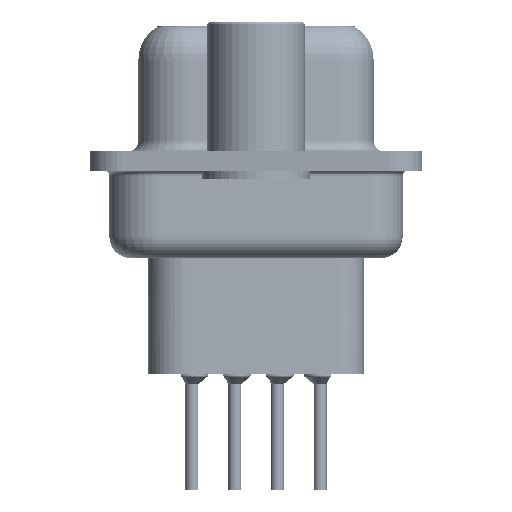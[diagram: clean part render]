
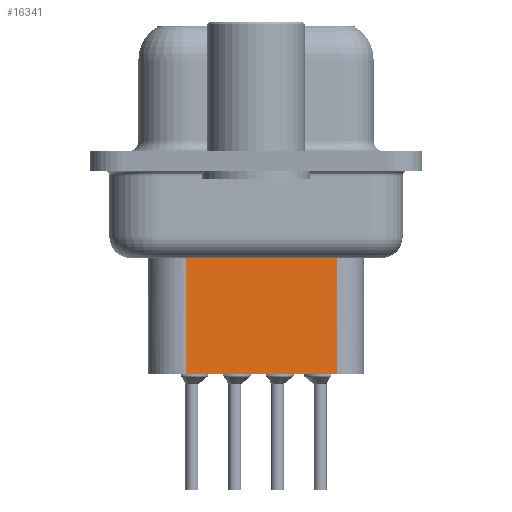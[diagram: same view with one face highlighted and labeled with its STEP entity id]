
A CAD part, left-side view. The second image highlights one B-rep face of the part: STEP entity #16341.
In plain terms, the highlighted planar face has unit normal (-0.985, -0.174, 0).
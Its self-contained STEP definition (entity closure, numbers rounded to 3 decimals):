
#1130 = EDGE_CURVE ( 'NONE', #27745, #7210, #40579, .T. ) ;
#2385 = DIRECTION ( 'NONE',  ( 0., 0., -1. ) ) ;
#2669 = EDGE_CURVE ( 'NONE', #3554, #58165, #57054, .T. ) ;
#2886 = LINE ( 'NONE', #30119, #45531 ) ;
#3420 = VECTOR ( 'NONE', #9770, 1000. ) ;
#3554 = VERTEX_POINT ( 'NONE', #17885 ) ;
#3828 = CARTESIAN_POINT ( 'NONE',  ( 4.453, 4.209, -3.975 ) ) ;
#4611 = FACE_OUTER_BOUND ( 'NONE', #24287, .T. ) ;
#5474 = PLANE ( 'NONE',  #20693 ) ;
#7210 = VERTEX_POINT ( 'NONE', #53471 ) ;
#7544 = ORIENTED_EDGE ( 'NONE', *, *, #25892, .T. ) ;
#9770 = DIRECTION ( 'NONE',  ( -0.174, 0.985, 0. ) ) ;
#10212 = CARTESIAN_POINT ( 'NONE',  ( 4.624, 3.24, -3.1 ) ) ;
#11851 = CARTESIAN_POINT ( 'NONE',  ( 4.624, 3.24, -3.1 ) ) ;
#13876 = ORIENTED_EDGE ( 'NONE', *, *, #1130, .F. ) ;
#16341 = ADVANCED_FACE ( 'NONE', ( #4611 ), #5474, .T. ) ;
#17885 = CARTESIAN_POINT ( 'NONE',  ( 5.858, -3.76, -3.975 ) ) ;
#20060 = DIRECTION ( 'NONE',  ( 0., 0., -1. ) ) ;
#20693 = AXIS2_PLACEMENT_3D ( 'NONE', #10212, #31832, #23549 ) ;
#23549 = DIRECTION ( 'NONE',  ( 0.174, -0.985, 0. ) ) ;
#24287 = EDGE_LOOP ( 'NONE', ( #37516, #40035, #7544, #13876 ) ) ;
#25892 = EDGE_CURVE ( 'NONE', #58165, #7210, #42059, .T. ) ;
#27745 = VERTEX_POINT ( 'NONE', #53079 ) ;
#30119 = CARTESIAN_POINT ( 'NONE',  ( 5.858, -3.76, -3.1 ) ) ;
#31832 = DIRECTION ( 'NONE',  ( -0.985, -0.174, 0. ) ) ;
#33166 = VECTOR ( 'NONE', #2385, 1000. ) ;
#33426 = CARTESIAN_POINT ( 'NONE',  ( 4.624, 3.24, -3.975 ) ) ;
#37516 = ORIENTED_EDGE ( 'NONE', *, *, #45650, .F. ) ;
#38808 = VECTOR ( 'NONE', #43807, 1000. ) ;
#40035 = ORIENTED_EDGE ( 'NONE', *, *, #2669, .T. ) ;
#40579 = LINE ( 'NONE', #45605, #3420 ) ;
#42059 = LINE ( 'NONE', #11851, #33166 ) ;
#43807 = DIRECTION ( 'NONE',  ( -0.174, 0.985, 0. ) ) ;
#45531 = VECTOR ( 'NONE', #20060, 1000. ) ;
#45605 = CARTESIAN_POINT ( 'NONE',  ( 4.624, 3.24, -9.85 ) ) ;
#45650 = EDGE_CURVE ( 'NONE', #3554, #27745, #2886, .T. ) ;
#53079 = CARTESIAN_POINT ( 'NONE',  ( 5.858, -3.76, -9.85 ) ) ;
#53471 = CARTESIAN_POINT ( 'NONE',  ( 4.624, 3.24, -9.85 ) ) ;
#57054 = LINE ( 'NONE', #3828, #38808 ) ;
#58165 = VERTEX_POINT ( 'NONE', #33426 ) ;
